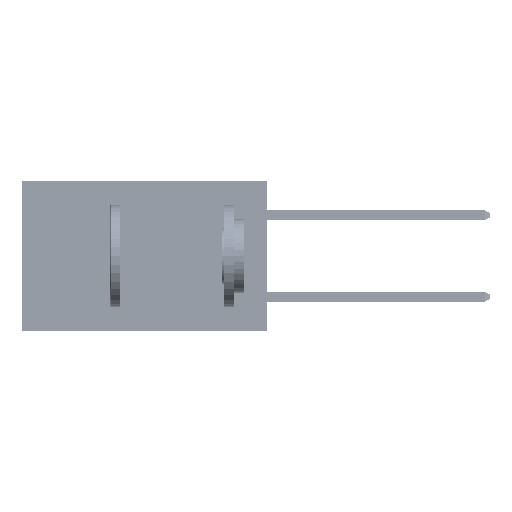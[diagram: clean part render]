
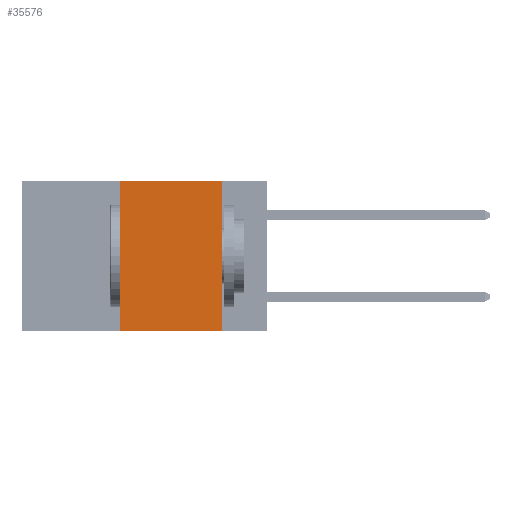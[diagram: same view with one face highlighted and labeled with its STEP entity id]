
A CAD part, left-side view. The second image highlights one B-rep face of the part: STEP entity #35576.
In plain terms, the highlighted planar face has unit normal (-1, 0, 0).
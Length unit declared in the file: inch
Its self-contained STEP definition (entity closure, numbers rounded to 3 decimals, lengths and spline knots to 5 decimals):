
#554 = CARTESIAN_POINT ( 'NONE',  ( 0., 0.11, 0. ) ) ;
#878 = ORIENTED_EDGE ( 'NONE', *, *, #27787, .F. ) ;
#2755 = CARTESIAN_POINT ( 'NONE',  ( 0., 0.11, 0. ) ) ;
#3020 = VECTOR ( 'NONE', #21503, 39.37008 ) ;
#12663 = DIRECTION ( 'NONE',  ( 0., -1., 0. ) ) ;
#12938 = CARTESIAN_POINT ( 'NONE',  ( 0., 0.36, -0.37 ) ) ;
#14249 = DIRECTION ( 'NONE',  ( 1., 0., 0. ) ) ;
#14770 = LINE ( 'NONE', #25354, #3020 ) ;
#15010 = LINE ( 'NONE', #35603, #35372 ) ;
#18114 = ORIENTED_EDGE ( 'NONE', *, *, #39838, .F. ) ;
#21503 = DIRECTION ( 'NONE',  ( 0., -1., 0. ) ) ;
#24503 = EDGE_CURVE ( 'NONE', #30533, #33982, #14770, .T. ) ;
#25354 = CARTESIAN_POINT ( 'NONE',  ( 0., 0.6, -0.37 ) ) ;
#27740 = LINE ( 'NONE', #30609, #36666 ) ;
#27787 = EDGE_CURVE ( 'NONE', #36403, #36772, #15010, .T. ) ;
#27814 = DIRECTION ( 'NONE',  ( 0., 0., -1. ) ) ;
#28296 = CARTESIAN_POINT ( 'NONE',  ( 0., 0.11, -0.37 ) ) ;
#29502 = PLANE ( 'NONE',  #41323 ) ;
#30533 = VERTEX_POINT ( 'NONE', #12938 ) ;
#30609 = CARTESIAN_POINT ( 'NONE',  ( 0., 0.36, 0. ) ) ;
#31906 = ORIENTED_EDGE ( 'NONE', *, *, #33084, .F. ) ;
#33084 = EDGE_CURVE ( 'NONE', #30533, #36403, #27740, .T. ) ;
#33888 = LINE ( 'NONE', #554, #45216 ) ;
#33982 = VERTEX_POINT ( 'NONE', #28296 ) ;
#34272 = ORIENTED_EDGE ( 'NONE', *, *, #24503, .T. ) ;
#34434 = DIRECTION ( 'NONE',  ( 0., 0., 1. ) ) ;
#35372 = VECTOR ( 'NONE', #12663, 39.37008 ) ;
#35576 = ADVANCED_FACE ( 'NONE', ( #43235 ), #29502, .F. ) ;
#35600 = CARTESIAN_POINT ( 'NONE',  ( 0., 0.36, 0. ) ) ;
#35603 = CARTESIAN_POINT ( 'NONE',  ( 0., 0.6, 0. ) ) ;
#36403 = VERTEX_POINT ( 'NONE', #35600 ) ;
#36666 = VECTOR ( 'NONE', #34434, 39.37008 ) ;
#36772 = VERTEX_POINT ( 'NONE', #2755 ) ;
#37160 = CARTESIAN_POINT ( 'NONE',  ( 0., 0.6, 0. ) ) ;
#39838 = EDGE_CURVE ( 'NONE', #36772, #33982, #33888, .T. ) ;
#40989 = DIRECTION ( 'NONE',  ( 0., 0., -1. ) ) ;
#41323 = AXIS2_PLACEMENT_3D ( 'NONE', #37160, #14249, #40989 ) ;
#43235 = FACE_OUTER_BOUND ( 'NONE', #45385, .T. ) ;
#45216 = VECTOR ( 'NONE', #27814, 39.37008 ) ;
#45385 = EDGE_LOOP ( 'NONE', ( #18114, #878, #31906, #34272 ) ) ;
